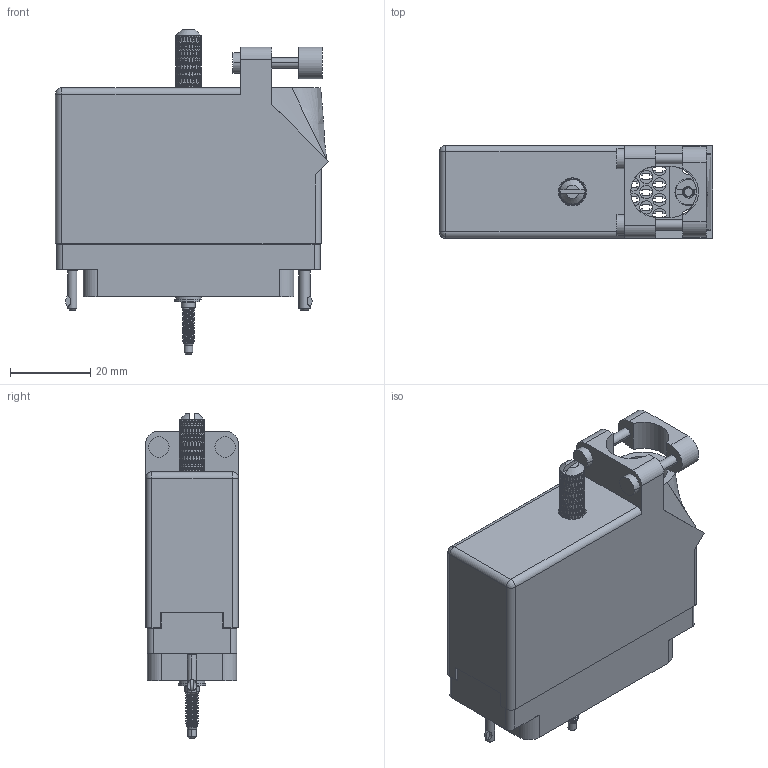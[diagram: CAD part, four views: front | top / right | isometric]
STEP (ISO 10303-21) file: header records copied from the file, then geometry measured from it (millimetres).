
FILE_DESCRIPTION (( 'STEP AP203' ), '1' );
FILE_NAME ('516-056-000-511.STEP', '2020-03-10T05:02:29', ( '' ), ( '' ), 'SwSTEP 2.0', 'SolidWorks 2016', '' );
FILE_SCHEMA (( 'CONFIG_CONTROL_DESIGN' ));
Length unit declared in the file: inch
Products named in the file (11): 516-253-035-100; 516-222-038-102_057; 516-222-038-102_056; 516-253-138-107; 516-251-035-100; 516-252-021-102_056; Actuating Screw Assy 038-056; 516-056-000-511; 516-250-038-111; 516-230-001_Plastic - 056 Top Entry; 516 Plug Insulator_056
Assembly tree (12 placements, depth 3):
  516-056-000-511
    516 Plug Insulator_056
    516-230-001_Plastic - 056 Top Entry
    516-252-021-102_056  x2
    516-222-038-102_056
    Actuating Screw Assy 038-056
      516-251-035-100
      516-253-035-100  x2
      516-253-138-107
      516-250-038-111
    516-222-038-102_057
Bounding box: 68.14 x 23.11 x 81.03 mm (x, y, z)
Volume: 26209.4 mm3; surface area: 35086.7 mm2
Topology: 11 solids, 11 shells, 2873 faces, 7250 edges, 4426 vertices
Faces by surface type: plane 1054, bspline 1045, cylinder 714, cone 54, torus 4, sphere 2
Entity records: 119328 total; most frequent: CARTESIAN_POINT 61413, ORIENTED_EDGE 14292, DIRECTION 9150, EDGE_CURVE 7146, VERTEX_POINT 4358, VECTOR 3070, LINE 3070, AXIS2_PLACEMENT_3D 3040
